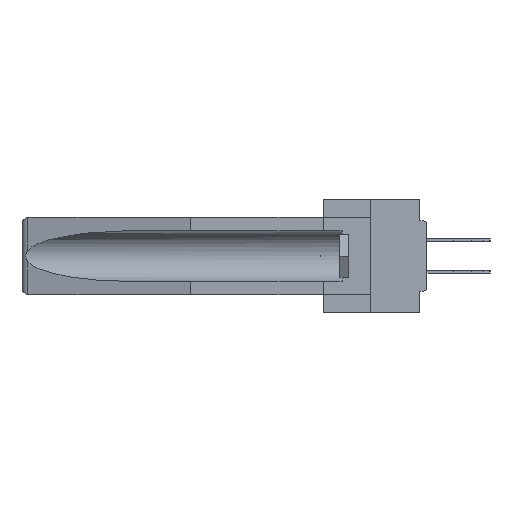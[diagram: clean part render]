
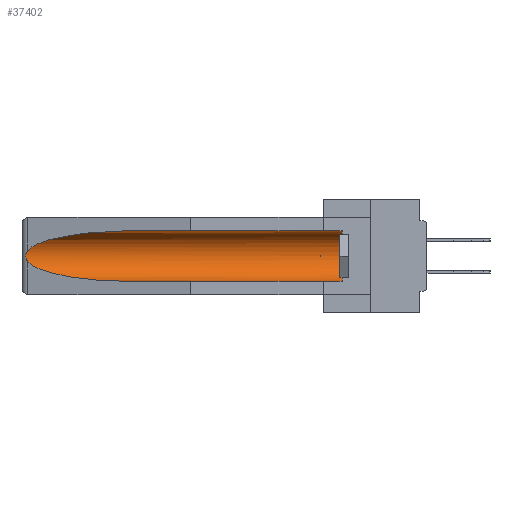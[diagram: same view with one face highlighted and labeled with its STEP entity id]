
A CAD part, left-side view. The second image highlights one B-rep face of the part: STEP entity #37402.
In plain terms, the highlighted cylindrical face has radius 2.857 mm (diameter 5.715 mm), a partial arc.
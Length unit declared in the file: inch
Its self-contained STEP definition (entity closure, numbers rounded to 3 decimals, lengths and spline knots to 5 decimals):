
#522 = CARTESIAN_POINT ( 'NONE',  ( 0.2675, 1.53308, -0.17534 ) ) ;
#561 = DIRECTION ( 'NONE',  ( 0., -1., 0. ) ) ;
#791 = AXIS2_PLACEMENT_3D ( 'NONE', #42162, #46213, #46038 ) ;
#970 = ORIENTED_EDGE ( 'NONE', *, *, #18589, .T. ) ;
#1584 = CARTESIAN_POINT ( 'NONE',  ( 0.26537, 1.52718, -0.19328 ) ) ;
#2396 = ORIENTED_EDGE ( 'NONE', *, *, #44116, .T. ) ;
#2607 = ORIENTED_EDGE ( 'NONE', *, *, #35257, .T. ) ;
#3119 = VERTEX_POINT ( 'NONE', #14610 ) ;
#4339 = ORIENTED_EDGE ( 'NONE', *, *, #26753, .F. ) ;
#4946 = CARTESIAN_POINT ( 'NONE',  ( 0.25451, 1.48313, -0.24835 ) ) ;
#5766 = VERTEX_POINT ( 'NONE', #40576 ) ;
#6333 = EDGE_CURVE ( 'NONE', #14205, #16465, #43056, .T. ) ;
#8061 = CARTESIAN_POINT ( 'NONE',  ( 0.26537, 1.52718, -0.19328 ) ) ;
#11185 = CARTESIAN_POINT ( 'NONE',  ( 0.155, 0.126, -0.284 ) ) ;
#11831 = CARTESIAN_POINT ( 'NONE',  ( 0.26537, 1.52718, -0.14972 ) ) ;
#12665 = EDGE_LOOP ( 'NONE', ( #2607, #43432, #30853, #4339, #970, #2396 ) ) ;
#13430 = CIRCLE ( 'NONE', #29249, 0.1125 ) ;
#14144 = EDGE_CURVE ( 'NONE', #16465, #5766, #34395, .T. ) ;
#14205 = VERTEX_POINT ( 'NONE', #16085 ) ;
#14610 = CARTESIAN_POINT ( 'NONE',  ( 0.155, 1.07973, -0.059 ) ) ;
#15013 = CARTESIAN_POINT ( 'NONE',  ( 0.26654, 1.53092, -0.15636 ) ) ;
#15387 = CARTESIAN_POINT ( 'NONE',  ( 0.155, 1.07973, -0.059 ) ) ;
#15572 = CARTESIAN_POINT ( 'NONE',  ( 0.155, -0.30754, -0.284 ) ) ;
#16085 = CARTESIAN_POINT ( 'NONE',  ( 0.26537, 1.52718, -0.14972 ) ) ;
#16465 = VERTEX_POINT ( 'NONE', #24293 ) ;
#16562 = CARTESIAN_POINT ( 'NONE',  ( 0.21114, 1.30732, -0.284 ) ) ;
#18544 = VERTEX_POINT ( 'NONE', #11185 ) ;
#18589 = EDGE_CURVE ( 'NONE', #18544, #36926, #13430, .T. ) ;
#20084 = CARTESIAN_POINT ( 'NONE',  ( 0.155, 1.07973, -0.284 ) ) ;
#22584 = CARTESIAN_POINT ( 'NONE',  ( 0.2675, 1.53308, -0.16763 ) ) ;
#22629 = CARTESIAN_POINT ( 'NONE',  ( 0.155, 0.126, -0.1715 ) ) ;
#22989 = DIRECTION ( 'NONE',  ( 0., 1., 0. ) ) ;
#23099 = CARTESIAN_POINT ( 'NONE',  ( 0.155, -0.30754, -0.059 ) ) ;
#23264 = DIRECTION ( 'NONE',  ( 0., 1., 0. ) ) ;
#24293 = CARTESIAN_POINT ( 'NONE',  ( 0.26537, 1.52718, -0.19328 ) ) ;
#25402 = LINE ( 'NONE', #23099, #39442 ) ;
#26226 = FACE_OUTER_BOUND ( 'NONE', #12665, .T. ) ;
#26311 = CARTESIAN_POINT ( 'NONE',  ( 0.155, 0.126, -0.059 ) ) ;
#26379 = DIRECTION ( 'NONE',  ( 0., 0., 1. ) ) ;
#26511 = CARTESIAN_POINT ( 'NONE',  ( 0.26655, 1.53094, -0.18657 ) ) ;
#26753 = EDGE_CURVE ( 'NONE', #18544, #5766, #36192, .T. ) ;
#27996 = CYLINDRICAL_SURFACE ( 'NONE', #791, 0.1125 ) ;
#29249 = AXIS2_PLACEMENT_3D ( 'NONE', #22629, #561, #26379 ) ;
#29950 = CARTESIAN_POINT ( 'NONE',  ( 0.2673, 1.5327, -0.16383 ) ) ;
#30276 = CARTESIAN_POINT ( 'NONE',  ( 0.26597, 1.5296, -0.19026 ) ) ;
#30853 = ORIENTED_EDGE ( 'NONE', *, *, #14144, .T. ) ;
#32960 =( BOUNDED_CURVE ( )  B_SPLINE_CURVE ( 3, ( #15387, #34055, #41320, #11831 ),
 .UNSPECIFIED., .F., .F. ) 
 B_SPLINE_CURVE_WITH_KNOTS ( ( 4, 4 ),
 ( 4.71239, 6.08839 ),
 .UNSPECIFIED. ) 
 CURVE ( )  GEOMETRIC_REPRESENTATION_ITEM ( )  RATIONAL_B_SPLINE_CURVE ( ( 1., 0.848, 0.848, 1. ) ) 
 REPRESENTATION_ITEM ( '' )  );
#34055 = CARTESIAN_POINT ( 'NONE',  ( 0.21114, 1.30732, -0.059 ) ) ;
#34395 =( BOUNDED_CURVE ( )  B_SPLINE_CURVE ( 3, ( #1584, #4946, #16562, #20084 ),
 .UNSPECIFIED., .F., .F. ) 
 B_SPLINE_CURVE_WITH_KNOTS ( ( 4, 4 ),
 ( 0.1948, 1.5708 ),
 .UNSPECIFIED. ) 
 CURVE ( )  GEOMETRIC_REPRESENTATION_ITEM ( )  RATIONAL_B_SPLINE_CURVE ( ( 1., 0.848, 0.848, 1. ) ) 
 REPRESENTATION_ITEM ( '' )  );
#35257 = EDGE_CURVE ( 'NONE', #3119, #14205, #32960, .T. ) ;
#36192 = LINE ( 'NONE', #15572, #40788 ) ;
#36926 = VERTEX_POINT ( 'NONE', #26311 ) ;
#37384 = CARTESIAN_POINT ( 'NONE',  ( 0.26537, 1.52718, -0.14972 ) ) ;
#37402 = ADVANCED_FACE ( 'NONE', ( #26226 ), #27996, .F. ) ;
#39442 = VECTOR ( 'NONE', #23264, 39.37008 ) ;
#40576 = CARTESIAN_POINT ( 'NONE',  ( 0.155, 1.07973, -0.284 ) ) ;
#40788 = VECTOR ( 'NONE', #22989, 39.37008 ) ;
#41258 = CARTESIAN_POINT ( 'NONE',  ( 0.26597, 1.52961, -0.15275 ) ) ;
#41320 = CARTESIAN_POINT ( 'NONE',  ( 0.25451, 1.48313, -0.09465 ) ) ;
#42162 = CARTESIAN_POINT ( 'NONE',  ( 0.155, -0.30754, -0.1715 ) ) ;
#43056 = B_SPLINE_CURVE_WITH_KNOTS ( 'NONE', 3,
 ( #37384, #41258, #15013, #29950, #22584, #522, #44991, #26511, #30276, #8061 ),
 .UNSPECIFIED., .F., .F.,
 ( 4, 2, 2, 2, 4 ),
 ( 0., 0.00029, 0.00058, 0.00087, 0.00117 ),
 .UNSPECIFIED. ) ;
#43432 = ORIENTED_EDGE ( 'NONE', *, *, #6333, .T. ) ;
#44116 = EDGE_CURVE ( 'NONE', #36926, #3119, #25402, .T. ) ;
#44991 = CARTESIAN_POINT ( 'NONE',  ( 0.2673, 1.53269, -0.17917 ) ) ;
#46038 = DIRECTION ( 'NONE',  ( 0., 0., 1. ) ) ;
#46213 = DIRECTION ( 'NONE',  ( 0., 1., 0. ) ) ;
